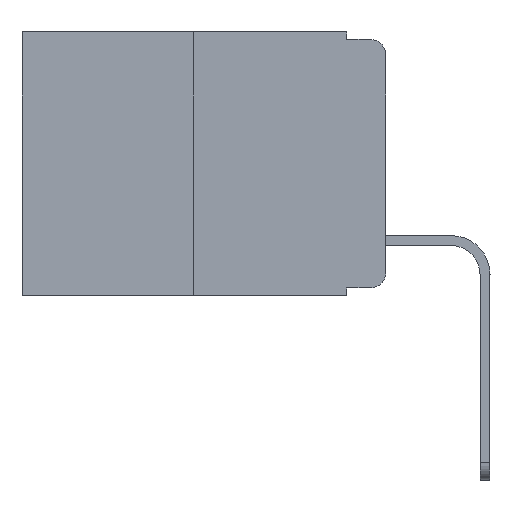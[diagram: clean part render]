
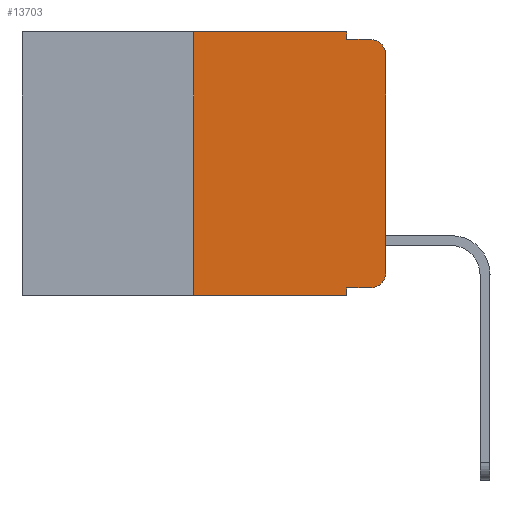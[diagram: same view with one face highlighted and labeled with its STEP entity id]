
A CAD part, left-side view. The second image highlights one B-rep face of the part: STEP entity #13703.
In plain terms, the highlighted planar face has unit normal (-1, 0, 0).
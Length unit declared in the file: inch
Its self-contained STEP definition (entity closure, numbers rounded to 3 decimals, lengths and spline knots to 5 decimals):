
#327 = VERTEX_POINT ( 'NONE', #14451 ) ;
#650 = AXIS2_PLACEMENT_3D ( 'NONE', #18534, #20136, #7481 ) ;
#819 = VECTOR ( 'NONE', #9010, 39.37008 ) ;
#833 = VERTEX_POINT ( 'NONE', #17804 ) ;
#972 = VECTOR ( 'NONE', #17486, 39.37008 ) ;
#1110 = LINE ( 'NONE', #10514, #5093 ) ;
#1156 = EDGE_CURVE ( 'NONE', #327, #4044, #22241, .T. ) ;
#1738 = CIRCLE ( 'NONE', #4017, 0.02 ) ;
#2471 = CARTESIAN_POINT ( 'NONE',  ( 0., 0.051, -0.343 ) ) ;
#2581 = DIRECTION ( 'NONE',  ( 0., 0., 1. ) ) ;
#3907 = CARTESIAN_POINT ( 'NONE',  ( 0., 0.02, -0.01 ) ) ;
#4017 = AXIS2_PLACEMENT_3D ( 'NONE', #8184, #6163, #20992 ) ;
#4044 = VERTEX_POINT ( 'NONE', #3907 ) ;
#4172 = VERTEX_POINT ( 'NONE', #2471 ) ;
#4495 = EDGE_CURVE ( 'NONE', #6294, #4172, #18965, .T. ) ;
#4716 = EDGE_CURVE ( 'NONE', #833, #4172, #10328, .T. ) ;
#5093 = VECTOR ( 'NONE', #6707, 39.37008 ) ;
#6163 = DIRECTION ( 'NONE',  ( -1., 0., 0. ) ) ;
#6176 = DIRECTION ( 'NONE',  ( 0., -1., 0. ) ) ;
#6294 = VERTEX_POINT ( 'NONE', #11676 ) ;
#6369 = LINE ( 'NONE', #8062, #22919 ) ;
#6707 = DIRECTION ( 'NONE',  ( 0., 0., 1. ) ) ;
#6917 = VECTOR ( 'NONE', #13591, 39.37008 ) ;
#7481 = DIRECTION ( 'NONE',  ( 0., 0., -1. ) ) ;
#7964 = CARTESIAN_POINT ( 'NONE',  ( 0., 0.25, 0. ) ) ;
#8062 = CARTESIAN_POINT ( 'NONE',  ( 0., 0.473, 0. ) ) ;
#8154 = VERTEX_POINT ( 'NONE', #15834 ) ;
#8184 = CARTESIAN_POINT ( 'NONE',  ( 0., 0.02, -0.313 ) ) ;
#8657 = CARTESIAN_POINT ( 'NONE',  ( 0., 0.473, 0. ) ) ;
#8922 = ORIENTED_EDGE ( 'NONE', *, *, #18302, .T. ) ;
#9010 = DIRECTION ( 'NONE',  ( 0., 0., -1. ) ) ;
#9415 = CARTESIAN_POINT ( 'NONE',  ( 0., 0.051, -0.333 ) ) ;
#9501 = DIRECTION ( 'NONE',  ( 0., -1., 0. ) ) ;
#9659 = FACE_OUTER_BOUND ( 'NONE', #17240, .T. ) ;
#10328 = LINE ( 'NONE', #23365, #22634 ) ;
#10415 = PLANE ( 'NONE',  #13814 ) ;
#10514 = CARTESIAN_POINT ( 'NONE',  ( 0., 0., 0. ) ) ;
#10825 = ORIENTED_EDGE ( 'NONE', *, *, #14205, .T. ) ;
#11347 = VECTOR ( 'NONE', #2581, 39.37008 ) ;
#11620 = ORIENTED_EDGE ( 'NONE', *, *, #21549, .F. ) ;
#11652 = CARTESIAN_POINT ( 'NONE',  ( 0., 0.02, -0.333 ) ) ;
#11676 = CARTESIAN_POINT ( 'NONE',  ( 0., 0.051, -0.333 ) ) ;
#11688 = LINE ( 'NONE', #9415, #17441 ) ;
#11739 = LINE ( 'NONE', #20712, #6917 ) ;
#12365 = ORIENTED_EDGE ( 'NONE', *, *, #1156, .T. ) ;
#12432 = EDGE_CURVE ( 'NONE', #23369, #21172, #1738, .T. ) ;
#12537 = VERTEX_POINT ( 'NONE', #23318 ) ;
#13097 = ORIENTED_EDGE ( 'NONE', *, *, #4716, .T. ) ;
#13591 = DIRECTION ( 'NONE',  ( 0., -1., 0. ) ) ;
#13703 = ADVANCED_FACE ( 'NONE', ( #9659 ), #10415, .F. ) ;
#13814 = AXIS2_PLACEMENT_3D ( 'NONE', #8657, #21284, #21603 ) ;
#14205 = EDGE_CURVE ( 'NONE', #21172, #327, #1110, .T. ) ;
#14348 = EDGE_CURVE ( 'NONE', #14876, #8154, #15340, .T. ) ;
#14451 = CARTESIAN_POINT ( 'NONE',  ( 0., 0., -0.03 ) ) ;
#14876 = VERTEX_POINT ( 'NONE', #19606 ) ;
#15340 = LINE ( 'NONE', #16200, #819 ) ;
#15524 = CARTESIAN_POINT ( 'NONE',  ( 0., 0., -0.313 ) ) ;
#15574 = ORIENTED_EDGE ( 'NONE', *, *, #12432, .T. ) ;
#15834 = CARTESIAN_POINT ( 'NONE',  ( 0., 0.051, -0.01 ) ) ;
#16200 = CARTESIAN_POINT ( 'NONE',  ( 0., 0.051, 0. ) ) ;
#17240 = EDGE_LOOP ( 'NONE', ( #10825, #12365, #19190, #17866, #11620, #18174, #13097, #19025, #8922, #15574 ) ) ;
#17441 = VECTOR ( 'NONE', #9501, 39.37008 ) ;
#17486 = DIRECTION ( 'NONE',  ( 0., 0., -1. ) ) ;
#17610 = EDGE_CURVE ( 'NONE', #8154, #4044, #11739, .T. ) ;
#17804 = CARTESIAN_POINT ( 'NONE',  ( 0., 0.25, -0.343 ) ) ;
#17866 = ORIENTED_EDGE ( 'NONE', *, *, #14348, .F. ) ;
#18174 = ORIENTED_EDGE ( 'NONE', *, *, #18369, .F. ) ;
#18302 = EDGE_CURVE ( 'NONE', #6294, #23369, #11688, .T. ) ;
#18369 = EDGE_CURVE ( 'NONE', #833, #12537, #23411, .T. ) ;
#18534 = CARTESIAN_POINT ( 'NONE',  ( 0., 0.02, -0.03 ) ) ;
#18965 = LINE ( 'NONE', #21157, #972 ) ;
#19025 = ORIENTED_EDGE ( 'NONE', *, *, #4495, .F. ) ;
#19190 = ORIENTED_EDGE ( 'NONE', *, *, #17610, .F. ) ;
#19606 = CARTESIAN_POINT ( 'NONE',  ( 0., 0.051, 0. ) ) ;
#19789 = DIRECTION ( 'NONE',  ( 0., -1., 0. ) ) ;
#20136 = DIRECTION ( 'NONE',  ( -1., 0., 0. ) ) ;
#20712 = CARTESIAN_POINT ( 'NONE',  ( 0., 0.051, -0.01 ) ) ;
#20992 = DIRECTION ( 'NONE',  ( 0., 0., -1. ) ) ;
#21157 = CARTESIAN_POINT ( 'NONE',  ( 0., 0.051, 0. ) ) ;
#21172 = VERTEX_POINT ( 'NONE', #15524 ) ;
#21284 = DIRECTION ( 'NONE',  ( 1., 0., 0. ) ) ;
#21549 = EDGE_CURVE ( 'NONE', #12537, #14876, #6369, .T. ) ;
#21603 = DIRECTION ( 'NONE',  ( 0., 0., -1. ) ) ;
#22241 = CIRCLE ( 'NONE', #650, 0.02 ) ;
#22634 = VECTOR ( 'NONE', #19789, 39.37008 ) ;
#22919 = VECTOR ( 'NONE', #6176, 39.37008 ) ;
#23318 = CARTESIAN_POINT ( 'NONE',  ( 0., 0.25, 0. ) ) ;
#23365 = CARTESIAN_POINT ( 'NONE',  ( 0., 0.473, -0.343 ) ) ;
#23369 = VERTEX_POINT ( 'NONE', #11652 ) ;
#23411 = LINE ( 'NONE', #7964, #11347 ) ;
